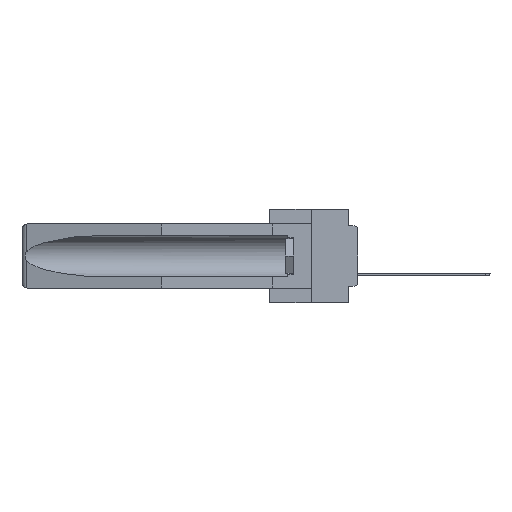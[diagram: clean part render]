
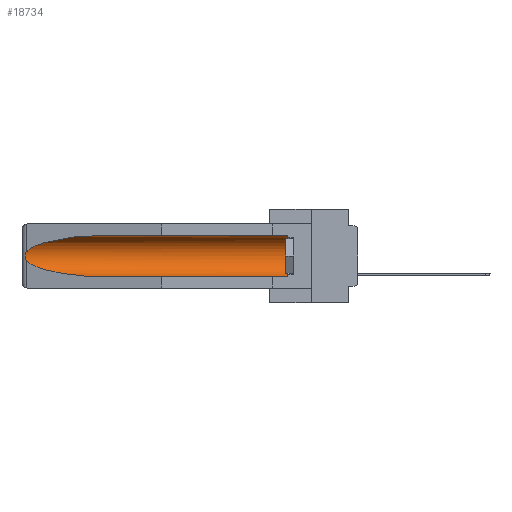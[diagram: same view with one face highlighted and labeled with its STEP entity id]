
A CAD part, left-side view. The second image highlights one B-rep face of the part: STEP entity #18734.
In plain terms, the highlighted cylindrical face has radius 2.857 mm (diameter 5.715 mm), a partial arc.
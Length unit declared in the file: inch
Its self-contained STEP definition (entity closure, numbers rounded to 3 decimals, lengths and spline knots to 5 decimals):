
#203 = ORIENTED_EDGE ( 'NONE', *, *, #10177, .T. ) ;
#552 = CARTESIAN_POINT ( 'NONE',  ( 0.155, -0.30754, -0.284 ) ) ;
#775 = EDGE_CURVE ( 'NONE', #7772, #11285, #14142, .T. ) ;
#809 = VERTEX_POINT ( 'NONE', #27745 ) ;
#842 = CARTESIAN_POINT ( 'NONE',  ( 0.155, 1.07973, -0.059 ) ) ;
#913 = ORIENTED_EDGE ( 'NONE', *, *, #3695, .T. ) ;
#1264 = CARTESIAN_POINT ( 'NONE',  ( 0.21114, 1.30732, -0.059 ) ) ;
#1363 = CARTESIAN_POINT ( 'NONE',  ( 0.26537, 1.52718, -0.14972 ) ) ;
#1653 = CARTESIAN_POINT ( 'NONE',  ( 0.155, 1.07973, -0.284 ) ) ;
#1898 = DIRECTION ( 'NONE',  ( 0., 0., 1. ) ) ;
#2504 = DIRECTION ( 'NONE',  ( 0., 1., 0. ) ) ;
#2609 = DIRECTION ( 'NONE',  ( 0., 0., 1. ) ) ;
#2692 = VECTOR ( 'NONE', #17512, 39.37008 ) ;
#3105 = VECTOR ( 'NONE', #18556, 39.37008 ) ;
#3390 = CARTESIAN_POINT ( 'NONE',  ( 0.25451, 1.48313, -0.09465 ) ) ;
#3695 = EDGE_CURVE ( 'NONE', #809, #18004, #26170, .T. ) ;
#3816 = CARTESIAN_POINT ( 'NONE',  ( 0.26537, 1.52718, -0.19328 ) ) ;
#5154 = CARTESIAN_POINT ( 'NONE',  ( 0.26537, 1.52718, -0.19328 ) ) ;
#5853 = CYLINDRICAL_SURFACE ( 'NONE', #22236, 0.1125 ) ;
#6506 = CARTESIAN_POINT ( 'NONE',  ( 0.25451, 1.48313, -0.24835 ) ) ;
#6701 = B_SPLINE_CURVE_WITH_KNOTS ( 'NONE', 3,
 ( #14989, #29968, #22424, #10199, #12728, #10304, #7739, #17703, #27379, #5154 ),
 .UNSPECIFIED., .F., .F.,
 ( 4, 2, 2, 2, 4 ),
 ( 0., 0.00029, 0.00058, 0.00087, 0.00117 ),
 .UNSPECIFIED. ) ;
#6813 = CARTESIAN_POINT ( 'NONE',  ( 0.21114, 1.30732, -0.284 ) ) ;
#7739 = CARTESIAN_POINT ( 'NONE',  ( 0.2673, 1.53269, -0.17917 ) ) ;
#7772 = VERTEX_POINT ( 'NONE', #3816 ) ;
#10177 = EDGE_CURVE ( 'NONE', #18004, #21642, #20439, .T. ) ;
#10199 = CARTESIAN_POINT ( 'NONE',  ( 0.2673, 1.5327, -0.16383 ) ) ;
#10304 = CARTESIAN_POINT ( 'NONE',  ( 0.2675, 1.53308, -0.17534 ) ) ;
#11285 = VERTEX_POINT ( 'NONE', #27444 ) ;
#11665 = CARTESIAN_POINT ( 'NONE',  ( 0.155, 0.126, -0.1715 ) ) ;
#12269 = CARTESIAN_POINT ( 'NONE',  ( 0.155, -0.30754, -0.1715 ) ) ;
#12728 = CARTESIAN_POINT ( 'NONE',  ( 0.2675, 1.53308, -0.16763 ) ) ;
#13132 = CARTESIAN_POINT ( 'NONE',  ( 0.26537, 1.52718, -0.14972 ) ) ;
#13391 = ORIENTED_EDGE ( 'NONE', *, *, #22585, .F. ) ;
#14100 = ORIENTED_EDGE ( 'NONE', *, *, #775, .T. ) ;
#14142 =( BOUNDED_CURVE ( )  B_SPLINE_CURVE ( 3, ( #16227, #6506, #6813, #1653 ),
 .UNSPECIFIED., .F., .F. ) 
 B_SPLINE_CURVE_WITH_KNOTS ( ( 4, 4 ),
 ( 0.1948, 1.5708 ),
 .UNSPECIFIED. ) 
 CURVE ( )  GEOMETRIC_REPRESENTATION_ITEM ( )  RATIONAL_B_SPLINE_CURVE ( ( 1., 0.848, 0.848, 1. ) ) 
 REPRESENTATION_ITEM ( '' )  );
#14865 = EDGE_LOOP ( 'NONE', ( #203, #20266, #14100, #13391, #26377, #913 ) ) ;
#14989 = CARTESIAN_POINT ( 'NONE',  ( 0.26537, 1.52718, -0.14972 ) ) ;
#16227 = CARTESIAN_POINT ( 'NONE',  ( 0.26537, 1.52718, -0.19328 ) ) ;
#17512 = DIRECTION ( 'NONE',  ( 0., 1., 0. ) ) ;
#17703 = CARTESIAN_POINT ( 'NONE',  ( 0.26655, 1.53094, -0.18657 ) ) ;
#18004 = VERTEX_POINT ( 'NONE', #842 ) ;
#18556 = DIRECTION ( 'NONE',  ( 0., 1., 0. ) ) ;
#18734 = ADVANCED_FACE ( 'NONE', ( #26225 ), #5853, .F. ) ;
#19360 = EDGE_CURVE ( 'NONE', #21642, #7772, #6701, .T. ) ;
#19392 = AXIS2_PLACEMENT_3D ( 'NONE', #11665, #28670, #1898 ) ;
#19782 = EDGE_CURVE ( 'NONE', #28392, #809, #30384, .T. ) ;
#20266 = ORIENTED_EDGE ( 'NONE', *, *, #19360, .T. ) ;
#20439 =( BOUNDED_CURVE ( )  B_SPLINE_CURVE ( 3, ( #30702, #1264, #3390, #13132 ),
 .UNSPECIFIED., .F., .F. ) 
 B_SPLINE_CURVE_WITH_KNOTS ( ( 4, 4 ),
 ( 4.71239, 6.08839 ),
 .UNSPECIFIED. ) 
 CURVE ( )  GEOMETRIC_REPRESENTATION_ITEM ( )  RATIONAL_B_SPLINE_CURVE ( ( 1., 0.848, 0.848, 1. ) ) 
 REPRESENTATION_ITEM ( '' )  );
#21642 = VERTEX_POINT ( 'NONE', #1363 ) ;
#22236 = AXIS2_PLACEMENT_3D ( 'NONE', #12269, #2504, #2609 ) ;
#22424 = CARTESIAN_POINT ( 'NONE',  ( 0.26654, 1.53092, -0.15636 ) ) ;
#22585 = EDGE_CURVE ( 'NONE', #28392, #11285, #27302, .T. ) ;
#26170 = LINE ( 'NONE', #30797, #3105 ) ;
#26225 = FACE_OUTER_BOUND ( 'NONE', #14865, .T. ) ;
#26377 = ORIENTED_EDGE ( 'NONE', *, *, #19782, .T. ) ;
#27302 = LINE ( 'NONE', #552, #2692 ) ;
#27379 = CARTESIAN_POINT ( 'NONE',  ( 0.26597, 1.5296, -0.19026 ) ) ;
#27444 = CARTESIAN_POINT ( 'NONE',  ( 0.155, 1.07973, -0.284 ) ) ;
#27745 = CARTESIAN_POINT ( 'NONE',  ( 0.155, 0.126, -0.059 ) ) ;
#28392 = VERTEX_POINT ( 'NONE', #28880 ) ;
#28670 = DIRECTION ( 'NONE',  ( 0., -1., 0. ) ) ;
#28880 = CARTESIAN_POINT ( 'NONE',  ( 0.155, 0.126, -0.284 ) ) ;
#29968 = CARTESIAN_POINT ( 'NONE',  ( 0.26597, 1.52961, -0.15275 ) ) ;
#30384 = CIRCLE ( 'NONE', #19392, 0.1125 ) ;
#30702 = CARTESIAN_POINT ( 'NONE',  ( 0.155, 1.07973, -0.059 ) ) ;
#30797 = CARTESIAN_POINT ( 'NONE',  ( 0.155, -0.30754, -0.059 ) ) ;
